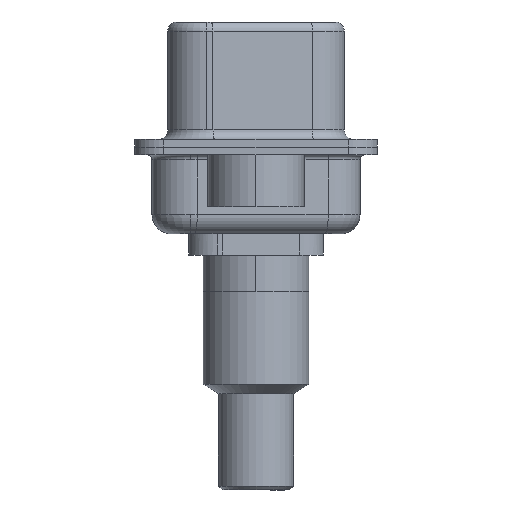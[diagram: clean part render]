
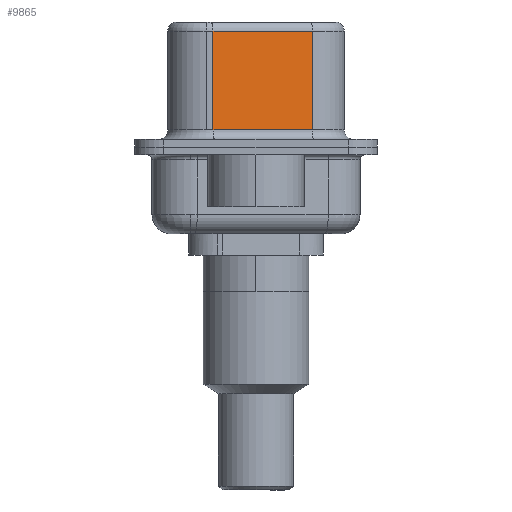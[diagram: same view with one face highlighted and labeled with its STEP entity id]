
A CAD part, left-side view. The second image highlights one B-rep face of the part: STEP entity #9865.
In plain terms, the highlighted planar face has unit normal (-0.985, -0.174, 0).
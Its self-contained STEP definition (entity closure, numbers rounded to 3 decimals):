
#925 = DIRECTION ( 'NONE',  ( 0.985, 0.174, 0. ) ) ;
#950 = DIRECTION ( 'NONE',  ( 0.174, -0.985, 0. ) ) ;
#1103 = CARTESIAN_POINT ( 'NONE',  ( 3.675, 2.233, 6.52 ) ) ;
#2171 = CARTESIAN_POINT ( 'NONE',  ( 4.585, -2.927, 0.9 ) ) ;
#3283 = CARTESIAN_POINT ( 'NONE',  ( 4.585, -2.927, 6.52 ) ) ;
#3412 = LINE ( 'NONE', #3283, #22849 ) ;
#3520 = DIRECTION ( 'NONE',  ( 0., 0., -1. ) ) ;
#3618 = VERTEX_POINT ( 'NONE', #2171 ) ;
#4245 = EDGE_LOOP ( 'NONE', ( #9199, #18021, #18984, #20483 ) ) ;
#4339 = EDGE_CURVE ( 'NONE', #15357, #16815, #10144, .T. ) ;
#4969 = EDGE_CURVE ( 'NONE', #16815, #5009, #21381, .T. ) ;
#5009 = VERTEX_POINT ( 'NONE', #22331 ) ;
#5088 = EDGE_CURVE ( 'NONE', #15357, #3618, #3412, .T. ) ;
#5232 = VECTOR ( 'NONE', #23032, 1000. ) ;
#6427 = FACE_OUTER_BOUND ( 'NONE', #4245, .T. ) ;
#9199 = ORIENTED_EDGE ( 'NONE', *, *, #5088, .F. ) ;
#9865 = ADVANCED_FACE ( 'NONE', ( #6427 ), #21579, .F. ) ;
#10144 = LINE ( 'NONE', #13612, #5232 ) ;
#11266 = DIRECTION ( 'NONE',  ( 0., 0., -1. ) ) ;
#11948 = CARTESIAN_POINT ( 'NONE',  ( 4.585, -2.927, 6.02 ) ) ;
#12144 = CARTESIAN_POINT ( 'NONE',  ( 4.585, -2.927, 6.52 ) ) ;
#13612 = CARTESIAN_POINT ( 'NONE',  ( 4.585, -2.927, 6.02 ) ) ;
#14049 = DIRECTION ( 'NONE',  ( -0.174, 0.985, 0. ) ) ;
#14277 = LINE ( 'NONE', #19715, #23749 ) ;
#15167 = VECTOR ( 'NONE', #11266, 1000. ) ;
#15357 = VERTEX_POINT ( 'NONE', #11948 ) ;
#16815 = VERTEX_POINT ( 'NONE', #19274 ) ;
#17408 = AXIS2_PLACEMENT_3D ( 'NONE', #12144, #925, #14049 ) ;
#18021 = ORIENTED_EDGE ( 'NONE', *, *, #4339, .T. ) ;
#18984 = ORIENTED_EDGE ( 'NONE', *, *, #4969, .T. ) ;
#19274 = CARTESIAN_POINT ( 'NONE',  ( 3.675, 2.233, 6.02 ) ) ;
#19715 = CARTESIAN_POINT ( 'NONE',  ( 4.585, -2.927, 0.9 ) ) ;
#20483 = ORIENTED_EDGE ( 'NONE', *, *, #23188, .T. ) ;
#21381 = LINE ( 'NONE', #1103, #15167 ) ;
#21579 = PLANE ( 'NONE',  #17408 ) ;
#22331 = CARTESIAN_POINT ( 'NONE',  ( 3.675, 2.233, 0.9 ) ) ;
#22849 = VECTOR ( 'NONE', #3520, 1000. ) ;
#23032 = DIRECTION ( 'NONE',  ( -0.174, 0.985, 0. ) ) ;
#23188 = EDGE_CURVE ( 'NONE', #5009, #3618, #14277, .T. ) ;
#23749 = VECTOR ( 'NONE', #950, 1000. ) ;
